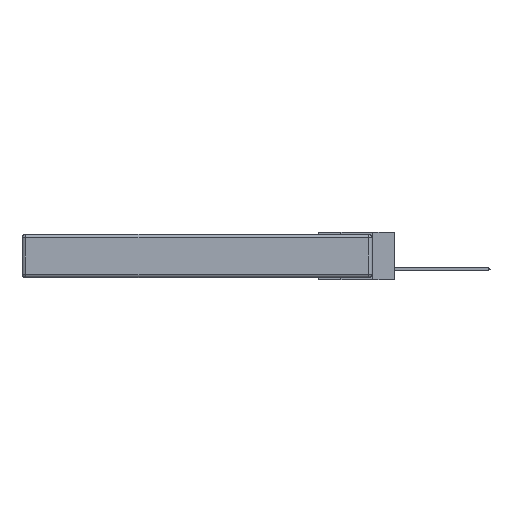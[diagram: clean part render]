
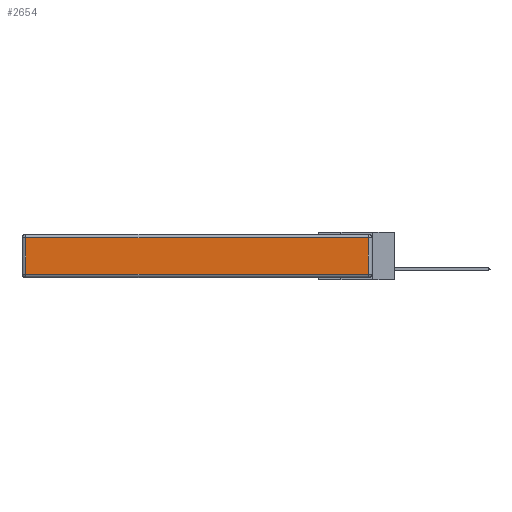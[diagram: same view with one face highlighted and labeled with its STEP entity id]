
A CAD part, left-side view. The second image highlights one B-rep face of the part: STEP entity #2654.
In plain terms, the highlighted planar face has unit normal (-1, 0, 0).
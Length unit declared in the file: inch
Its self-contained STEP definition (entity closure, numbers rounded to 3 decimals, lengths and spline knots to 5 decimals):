
#883 = DIRECTION ( 'NONE',  ( 0., 0., 1. ) ) ;
#1813 = CARTESIAN_POINT ( 'NONE',  ( 0., 0., -0.313 ) ) ;
#2144 = EDGE_CURVE ( 'NONE', #12350, #14303, #29429, .T. ) ;
#2654 = ADVANCED_FACE ( 'NONE', ( #27546 ), #29980, .T. ) ;
#3790 = DIRECTION ( 'NONE',  ( 0., -1., 0. ) ) ;
#4574 = CARTESIAN_POINT ( 'NONE',  ( 0., 2.72, -0.03 ) ) ;
#5057 = LINE ( 'NONE', #22717, #18515 ) ;
#6026 = CARTESIAN_POINT ( 'NONE',  ( 0., 0., -0.343 ) ) ;
#6087 = DIRECTION ( 'NONE',  ( 0., 1., 0. ) ) ;
#6707 = VECTOR ( 'NONE', #18331, 39.37008 ) ;
#7449 = CARTESIAN_POINT ( 'NONE',  ( 0., 0.03, -0.03 ) ) ;
#7859 = CARTESIAN_POINT ( 'NONE',  ( 0., 0.03, -0.343 ) ) ;
#9141 = LINE ( 'NONE', #7859, #25150 ) ;
#9331 = CARTESIAN_POINT ( 'NONE',  ( 0., 0.03, -0.313 ) ) ;
#11129 = LINE ( 'NONE', #1813, #20106 ) ;
#12350 = VERTEX_POINT ( 'NONE', #4574 ) ;
#12638 = EDGE_CURVE ( 'NONE', #28103, #12350, #5057, .T. ) ;
#13085 = ORIENTED_EDGE ( 'NONE', *, *, #21018, .T. ) ;
#14154 = CARTESIAN_POINT ( 'NONE',  ( 0., 2.72, -0.313 ) ) ;
#14303 = VERTEX_POINT ( 'NONE', #14154 ) ;
#15207 = AXIS2_PLACEMENT_3D ( 'NONE', #6026, #22871, #25320 ) ;
#16073 = VERTEX_POINT ( 'NONE', #9331 ) ;
#18331 = DIRECTION ( 'NONE',  ( 0., 0., -1. ) ) ;
#18515 = VECTOR ( 'NONE', #6087, 39.37008 ) ;
#20106 = VECTOR ( 'NONE', #3790, 39.37008 ) ;
#20365 = ORIENTED_EDGE ( 'NONE', *, *, #2144, .T. ) ;
#21018 = EDGE_CURVE ( 'NONE', #14303, #16073, #11129, .T. ) ;
#21289 = ORIENTED_EDGE ( 'NONE', *, *, #27016, .T. ) ;
#22717 = CARTESIAN_POINT ( 'NONE',  ( 0., 2.75, -0.03 ) ) ;
#22753 = ORIENTED_EDGE ( 'NONE', *, *, #12638, .T. ) ;
#22871 = DIRECTION ( 'NONE',  ( -1., 0., 0. ) ) ;
#25128 = EDGE_LOOP ( 'NONE', ( #13085, #21289, #22753, #20365 ) ) ;
#25150 = VECTOR ( 'NONE', #883, 39.37008 ) ;
#25320 = DIRECTION ( 'NONE',  ( 0., 0., 1. ) ) ;
#27016 = EDGE_CURVE ( 'NONE', #16073, #28103, #9141, .T. ) ;
#27546 = FACE_OUTER_BOUND ( 'NONE', #25128, .T. ) ;
#28103 = VERTEX_POINT ( 'NONE', #7449 ) ;
#29429 = LINE ( 'NONE', #30127, #6707 ) ;
#29980 = PLANE ( 'NONE',  #15207 ) ;
#30127 = CARTESIAN_POINT ( 'NONE',  ( 0., 2.72, -0.343 ) ) ;
